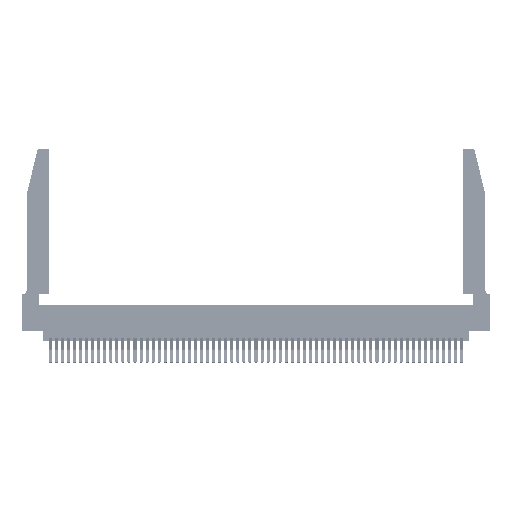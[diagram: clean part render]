
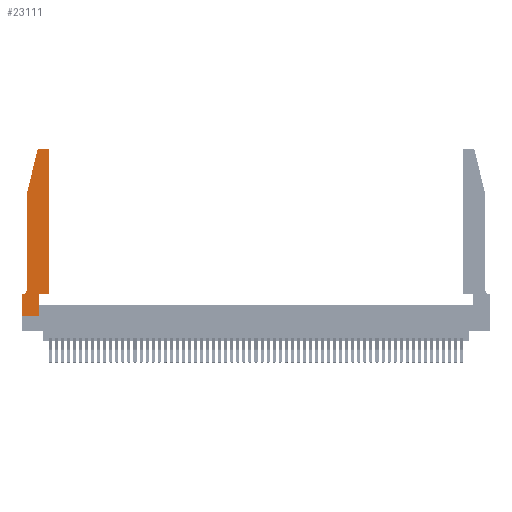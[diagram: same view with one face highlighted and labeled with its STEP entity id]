
A CAD part, top view. The second image highlights one B-rep face of the part: STEP entity #23111.
In plain terms, the highlighted planar face has unit normal (0, 0, 1).
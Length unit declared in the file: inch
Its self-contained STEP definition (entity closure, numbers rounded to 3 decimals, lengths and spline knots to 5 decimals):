
#751 = VECTOR ( 'NONE', #15444, 39.37008 ) ;
#3109 = VERTEX_POINT ( 'NONE', #16736 ) ;
#3577 = CARTESIAN_POINT ( 'NONE',  ( 0.2865, 0., 0.37 ) ) ;
#4018 = LINE ( 'NONE', #33471, #46938 ) ;
#4020 = LINE ( 'NONE', #50736, #51630 ) ;
#4284 = VERTEX_POINT ( 'NONE', #22071 ) ;
#4575 = ORIENTED_EDGE ( 'NONE', *, *, #28998, .T. ) ;
#5992 = VECTOR ( 'NONE', #26040, 39.37008 ) ;
#6985 = CARTESIAN_POINT ( 'NONE',  ( 0., 0., 0.37 ) ) ;
#7006 = CARTESIAN_POINT ( 'NONE',  ( 0.2865, 0.35, 0.37 ) ) ;
#7462 = AXIS2_PLACEMENT_3D ( 'NONE', #14791, #48665, #14975 ) ;
#8298 = CARTESIAN_POINT ( 'NONE',  ( 0., 0.35, 0.37 ) ) ;
#8299 = CARTESIAN_POINT ( 'NONE',  ( 0.2605, 2.75, 0.37 ) ) ;
#8846 = DIRECTION ( 'NONE',  ( 1., 0., 0. ) ) ;
#9087 = CARTESIAN_POINT ( 'NONE',  ( 0., 0., 0.37 ) ) ;
#9172 = CARTESIAN_POINT ( 'NONE',  ( 0.4505, 2.72, 0.37 ) ) ;
#9728 = CIRCLE ( 'NONE', #7462, 0.07 ) ;
#11312 = CARTESIAN_POINT ( 'NONE',  ( 0.25487, 2.72718, 0.37 ) ) ;
#11320 = CARTESIAN_POINT ( 'NONE',  ( 0.0055, 0.35, 0.37 ) ) ;
#11442 = VERTEX_POINT ( 'NONE', #11312 ) ;
#11647 = CARTESIAN_POINT ( 'NONE',  ( 0.0755, 2., 0.37 ) ) ;
#12102 = LINE ( 'NONE', #11647, #48933 ) ;
#12533 = CARTESIAN_POINT ( 'NONE',  ( 0.4505, 0.35, 0.37 ) ) ;
#13319 = CARTESIAN_POINT ( 'NONE',  ( 0.4505, 0.35, 0.37 ) ) ;
#14005 = EDGE_CURVE ( 'NONE', #3109, #47931, #4018, .T. ) ;
#14124 = ORIENTED_EDGE ( 'NONE', *, *, #34445, .T. ) ;
#14349 = AXIS2_PLACEMENT_3D ( 'NONE', #50897, #54477, #55035 ) ;
#14791 = CARTESIAN_POINT ( 'NONE',  ( 0.0055, 0.42, 0.37 ) ) ;
#14975 = DIRECTION ( 'NONE',  ( -1., 0., 0. ) ) ;
#15444 = DIRECTION ( 'NONE',  ( 0., -1., 0. ) ) ;
#15549 = LINE ( 'NONE', #33044, #751 ) ;
#16736 = CARTESIAN_POINT ( 'NONE',  ( 0.0755, 2., 0.37 ) ) ;
#16976 = VERTEX_POINT ( 'NONE', #3577 ) ;
#17347 = DIRECTION ( 'NONE',  ( 1., 0., 0. ) ) ;
#17473 = EDGE_CURVE ( 'NONE', #47544, #31370, #19725, .T. ) ;
#19108 = VERTEX_POINT ( 'NONE', #24273 ) ;
#19486 = ORIENTED_EDGE ( 'NONE', *, *, #34604, .T. ) ;
#19725 = CIRCLE ( 'NONE', #52676, 0.03 ) ;
#20251 = CARTESIAN_POINT ( 'NONE',  ( 0., 0.35, 0.37 ) ) ;
#20756 = DIRECTION ( 'NONE',  ( 0., -1., 0. ) ) ;
#22071 = CARTESIAN_POINT ( 'NONE',  ( 0.284, 2.75, 0.37 ) ) ;
#23111 = ADVANCED_FACE ( 'NONE', ( #46634 ), #34514, .T. ) ;
#24273 = CARTESIAN_POINT ( 'NONE',  ( 0.2865, 0.35, 0.37 ) ) ;
#24328 = VERTEX_POINT ( 'NONE', #11320 ) ;
#24991 = CARTESIAN_POINT ( 'NONE',  ( 0.4205, 2.75, 0.37 ) ) ;
#25826 = ORIENTED_EDGE ( 'NONE', *, *, #46880, .T. ) ;
#25834 = DIRECTION ( 'NONE',  ( 1., 0., 0. ) ) ;
#26040 = DIRECTION ( 'NONE',  ( 0., 1., 0. ) ) ;
#28459 = LINE ( 'NONE', #12533, #34450 ) ;
#28501 = ORIENTED_EDGE ( 'NONE', *, *, #34303, .T. ) ;
#28524 = LINE ( 'NONE', #8299, #44538 ) ;
#28998 = EDGE_CURVE ( 'NONE', #16976, #19108, #29921, .T. ) ;
#29921 = LINE ( 'NONE', #7006, #31251 ) ;
#29967 = EDGE_CURVE ( 'NONE', #4284, #11442, #43876, .T. ) ;
#30152 = EDGE_CURVE ( 'NONE', #19108, #34357, #28459, .T. ) ;
#30704 = EDGE_LOOP ( 'NONE', ( #25826, #52898, #28501, #36738, #32755, #14124, #33162, #48499, #4575, #43374, #19486, #51291 ) ) ;
#31251 = VECTOR ( 'NONE', #41474, 39.37008 ) ;
#31370 = VERTEX_POINT ( 'NONE', #24991 ) ;
#31692 = VECTOR ( 'NONE', #17347, 39.37008 ) ;
#32755 = ORIENTED_EDGE ( 'NONE', *, *, #38806, .T. ) ;
#33044 = CARTESIAN_POINT ( 'NONE',  ( 0., 0., 0.37 ) ) ;
#33162 = ORIENTED_EDGE ( 'NONE', *, *, #55450, .T. ) ;
#33412 = EDGE_CURVE ( 'NONE', #51490, #16976, #40295, .T. ) ;
#33471 = CARTESIAN_POINT ( 'NONE',  ( 0.0755, 2., 0.37 ) ) ;
#33764 = DIRECTION ( 'NONE',  ( -1., 0., 0. ) ) ;
#34303 = EDGE_CURVE ( 'NONE', #11442, #3109, #12102, .T. ) ;
#34357 = VERTEX_POINT ( 'NONE', #37100 ) ;
#34445 = EDGE_CURVE ( 'NONE', #24328, #37406, #4020, .T. ) ;
#34450 = VECTOR ( 'NONE', #25834, 39.37008 ) ;
#34514 = PLANE ( 'NONE',  #51016 ) ;
#34604 = EDGE_CURVE ( 'NONE', #34357, #47544, #35511, .T. ) ;
#35511 = LINE ( 'NONE', #13319, #5992 ) ;
#36738 = ORIENTED_EDGE ( 'NONE', *, *, #14005, .T. ) ;
#37100 = CARTESIAN_POINT ( 'NONE',  ( 0.4505, 0.35, 0.37 ) ) ;
#37406 = VERTEX_POINT ( 'NONE', #20251 ) ;
#37676 = CARTESIAN_POINT ( 'NONE',  ( 0.0755, 0.42, 0.37 ) ) ;
#38444 = DIRECTION ( 'NONE',  ( 0., 0., 1. ) ) ;
#38806 = EDGE_CURVE ( 'NONE', #47931, #24328, #9728, .T. ) ;
#40295 = LINE ( 'NONE', #9087, #31692 ) ;
#41474 = DIRECTION ( 'NONE',  ( 0., 1., 0. ) ) ;
#43374 = ORIENTED_EDGE ( 'NONE', *, *, #30152, .T. ) ;
#43876 = CIRCLE ( 'NONE', #14349, 0.03 ) ;
#44538 = VECTOR ( 'NONE', #33764, 39.37008 ) ;
#45329 = DIRECTION ( 'NONE',  ( -0.239, -0.971, 0. ) ) ;
#46634 = FACE_OUTER_BOUND ( 'NONE', #30704, .T. ) ;
#46880 = EDGE_CURVE ( 'NONE', #31370, #4284, #28524, .T. ) ;
#46938 = VECTOR ( 'NONE', #20756, 39.37008 ) ;
#47243 = CARTESIAN_POINT ( 'NONE',  ( 0.4205, 2.72, 0.37 ) ) ;
#47544 = VERTEX_POINT ( 'NONE', #9172 ) ;
#47931 = VERTEX_POINT ( 'NONE', #37676 ) ;
#48499 = ORIENTED_EDGE ( 'NONE', *, *, #33412, .T. ) ;
#48665 = DIRECTION ( 'NONE',  ( 0., 0., -1. ) ) ;
#48933 = VECTOR ( 'NONE', #45329, 39.37008 ) ;
#50736 = CARTESIAN_POINT ( 'NONE',  ( 0.0755, 0.35, 0.37 ) ) ;
#50897 = CARTESIAN_POINT ( 'NONE',  ( 0.284, 2.72, 0.37 ) ) ;
#51016 = AXIS2_PLACEMENT_3D ( 'NONE', #8298, #38444, #8846 ) ;
#51291 = ORIENTED_EDGE ( 'NONE', *, *, #17473, .T. ) ;
#51377 = DIRECTION ( 'NONE',  ( 1., 0., 0. ) ) ;
#51490 = VERTEX_POINT ( 'NONE', #6985 ) ;
#51630 = VECTOR ( 'NONE', #55069, 39.37008 ) ;
#52320 = DIRECTION ( 'NONE',  ( 0., 0., 1. ) ) ;
#52676 = AXIS2_PLACEMENT_3D ( 'NONE', #47243, #52320, #51377 ) ;
#52898 = ORIENTED_EDGE ( 'NONE', *, *, #29967, .T. ) ;
#54477 = DIRECTION ( 'NONE',  ( 0., 0., 1. ) ) ;
#55035 = DIRECTION ( 'NONE',  ( 1., 0., 0. ) ) ;
#55069 = DIRECTION ( 'NONE',  ( -1., 0., 0. ) ) ;
#55450 = EDGE_CURVE ( 'NONE', #37406, #51490, #15549, .T. ) ;
